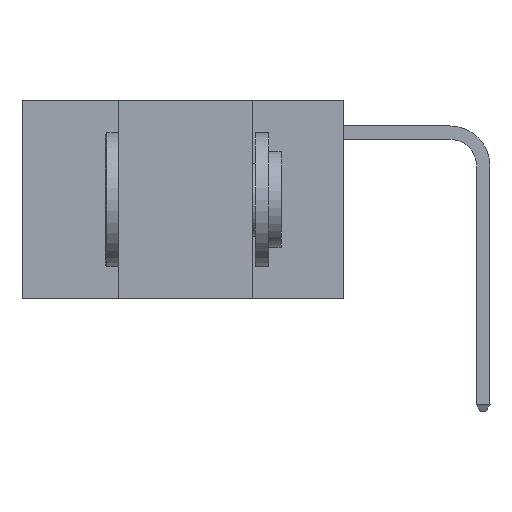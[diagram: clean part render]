
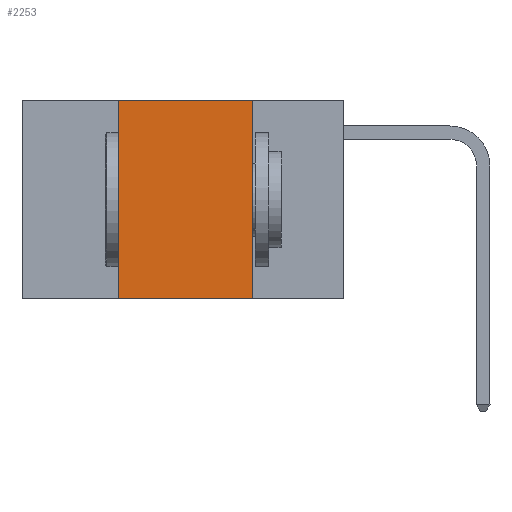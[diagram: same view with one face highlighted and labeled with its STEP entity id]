
A CAD part, left-side view. The second image highlights one B-rep face of the part: STEP entity #2253.
In plain terms, the highlighted planar face has unit normal (-1, 0, 0).
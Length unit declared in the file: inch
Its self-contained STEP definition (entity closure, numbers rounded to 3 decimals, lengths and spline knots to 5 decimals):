
#292 = LINE ( 'NONE', #5100, #22505 ) ;
#713 = DIRECTION ( 'NONE',  ( 0., -1., 0. ) ) ;
#950 = DIRECTION ( 'NONE',  ( 0., 0., 1. ) ) ;
#1839 = VECTOR ( 'NONE', #6232, 39.37008 ) ;
#2056 = CARTESIAN_POINT ( 'NONE',  ( 0., 0.6, -0.37 ) ) ;
#2253 = ADVANCED_FACE ( 'NONE', ( #10951 ), #16522, .F. ) ;
#3433 = ORIENTED_EDGE ( 'NONE', *, *, #25789, .F. ) ;
#3990 = DIRECTION ( 'NONE',  ( 1., 0., 0. ) ) ;
#5100 = CARTESIAN_POINT ( 'NONE',  ( 0., 0.17, 0. ) ) ;
#5648 = EDGE_CURVE ( 'NONE', #25045, #14546, #19604, .T. ) ;
#6232 = DIRECTION ( 'NONE',  ( 0., -1., 0. ) ) ;
#7395 = VERTEX_POINT ( 'NONE', #16837 ) ;
#8489 = VECTOR ( 'NONE', #713, 39.37008 ) ;
#8830 = VECTOR ( 'NONE', #950, 39.37008 ) ;
#10596 = EDGE_LOOP ( 'NONE', ( #3433, #14536, #15182, #26233 ) ) ;
#10825 = EDGE_CURVE ( 'NONE', #7395, #12731, #12899, .T. ) ;
#10951 = FACE_OUTER_BOUND ( 'NONE', #10596, .T. ) ;
#12600 = CARTESIAN_POINT ( 'NONE',  ( 0., 0.42, 0. ) ) ;
#12731 = VERTEX_POINT ( 'NONE', #16467 ) ;
#12899 = LINE ( 'NONE', #2056, #1839 ) ;
#14536 = ORIENTED_EDGE ( 'NONE', *, *, #5648, .F. ) ;
#14546 = VERTEX_POINT ( 'NONE', #22000 ) ;
#15182 = ORIENTED_EDGE ( 'NONE', *, *, #20631, .F. ) ;
#16467 = CARTESIAN_POINT ( 'NONE',  ( 0., 0.17, -0.37 ) ) ;
#16522 = PLANE ( 'NONE',  #17054 ) ;
#16837 = CARTESIAN_POINT ( 'NONE',  ( 0., 0.42, -0.37 ) ) ;
#17054 = AXIS2_PLACEMENT_3D ( 'NONE', #24761, #3990, #18637 ) ;
#18637 = DIRECTION ( 'NONE',  ( 0., 0., -1. ) ) ;
#19604 = LINE ( 'NONE', #23572, #8489 ) ;
#19723 = DIRECTION ( 'NONE',  ( 0., 0., -1. ) ) ;
#20631 = EDGE_CURVE ( 'NONE', #7395, #25045, #20636, .T. ) ;
#20636 = LINE ( 'NONE', #23806, #8830 ) ;
#22000 = CARTESIAN_POINT ( 'NONE',  ( 0., 0.17, 0. ) ) ;
#22505 = VECTOR ( 'NONE', #19723, 39.37008 ) ;
#23572 = CARTESIAN_POINT ( 'NONE',  ( 0., 0.6, 0. ) ) ;
#23806 = CARTESIAN_POINT ( 'NONE',  ( 0., 0.42, 0. ) ) ;
#24761 = CARTESIAN_POINT ( 'NONE',  ( 0., 0.6, 0. ) ) ;
#25045 = VERTEX_POINT ( 'NONE', #12600 ) ;
#25789 = EDGE_CURVE ( 'NONE', #14546, #12731, #292, .T. ) ;
#26233 = ORIENTED_EDGE ( 'NONE', *, *, #10825, .T. ) ;
